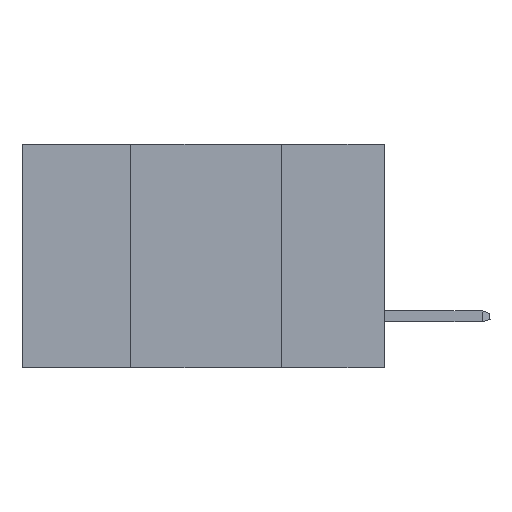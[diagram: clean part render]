
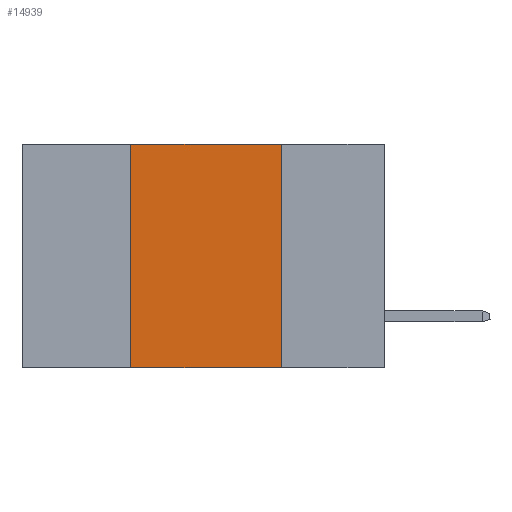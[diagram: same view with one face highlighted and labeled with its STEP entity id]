
A CAD part, left-side view. The second image highlights one B-rep face of the part: STEP entity #14939.
In plain terms, the highlighted planar face has unit normal (-1, 0, 0).
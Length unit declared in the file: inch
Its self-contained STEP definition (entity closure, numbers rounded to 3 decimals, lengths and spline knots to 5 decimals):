
#390 = DIRECTION ( 'NONE',  ( 0., 0., -1. ) ) ;
#752 = CARTESIAN_POINT ( 'NONE',  ( 0., 0.6, 0. ) ) ;
#1614 = EDGE_LOOP ( 'NONE', ( #21079, #11692, #20785, #9456 ) ) ;
#2206 = AXIS2_PLACEMENT_3D ( 'NONE', #14003, #19750, #15979 ) ;
#2300 = CARTESIAN_POINT ( 'NONE',  ( 0., 0.6, -0.37 ) ) ;
#2815 = LINE ( 'NONE', #23054, #15890 ) ;
#4247 = CARTESIAN_POINT ( 'NONE',  ( 0., 0.42, -0.37 ) ) ;
#4285 = VERTEX_POINT ( 'NONE', #16015 ) ;
#6378 = VERTEX_POINT ( 'NONE', #20523 ) ;
#6740 = DIRECTION ( 'NONE',  ( 0., -1., 0. ) ) ;
#6772 = FACE_OUTER_BOUND ( 'NONE', #1614, .T. ) ;
#7724 = EDGE_CURVE ( 'NONE', #4285, #14689, #2815, .T. ) ;
#8764 = LINE ( 'NONE', #752, #12882 ) ;
#9456 = ORIENTED_EDGE ( 'NONE', *, *, #21856, .T. ) ;
#10110 = VERTEX_POINT ( 'NONE', #4247 ) ;
#11015 = EDGE_CURVE ( 'NONE', #6378, #4285, #8764, .T. ) ;
#11692 = ORIENTED_EDGE ( 'NONE', *, *, #11015, .F. ) ;
#12292 = LINE ( 'NONE', #2300, #23625 ) ;
#12882 = VECTOR ( 'NONE', #6740, 39.37008 ) ;
#14003 = CARTESIAN_POINT ( 'NONE',  ( 0., 0.6, 0. ) ) ;
#14689 = VERTEX_POINT ( 'NONE', #18802 ) ;
#14939 = ADVANCED_FACE ( 'NONE', ( #6772 ), #21570, .F. ) ;
#15890 = VECTOR ( 'NONE', #390, 39.37008 ) ;
#15979 = DIRECTION ( 'NONE',  ( 0., 0., -1. ) ) ;
#16015 = CARTESIAN_POINT ( 'NONE',  ( 0., 0.17, 0. ) ) ;
#16650 = CARTESIAN_POINT ( 'NONE',  ( 0., 0.42, 0. ) ) ;
#17773 = VECTOR ( 'NONE', #24648, 39.37008 ) ;
#18802 = CARTESIAN_POINT ( 'NONE',  ( 0., 0.17, -0.37 ) ) ;
#19530 = EDGE_CURVE ( 'NONE', #10110, #6378, #24042, .T. ) ;
#19750 = DIRECTION ( 'NONE',  ( 1., 0., 0. ) ) ;
#20523 = CARTESIAN_POINT ( 'NONE',  ( 0., 0.42, 0. ) ) ;
#20785 = ORIENTED_EDGE ( 'NONE', *, *, #19530, .F. ) ;
#21079 = ORIENTED_EDGE ( 'NONE', *, *, #7724, .F. ) ;
#21570 = PLANE ( 'NONE',  #2206 ) ;
#21856 = EDGE_CURVE ( 'NONE', #10110, #14689, #12292, .T. ) ;
#22908 = DIRECTION ( 'NONE',  ( 0., -1., 0. ) ) ;
#23054 = CARTESIAN_POINT ( 'NONE',  ( 0., 0.17, 0. ) ) ;
#23625 = VECTOR ( 'NONE', #22908, 39.37008 ) ;
#24042 = LINE ( 'NONE', #16650, #17773 ) ;
#24648 = DIRECTION ( 'NONE',  ( 0., 0., 1. ) ) ;
